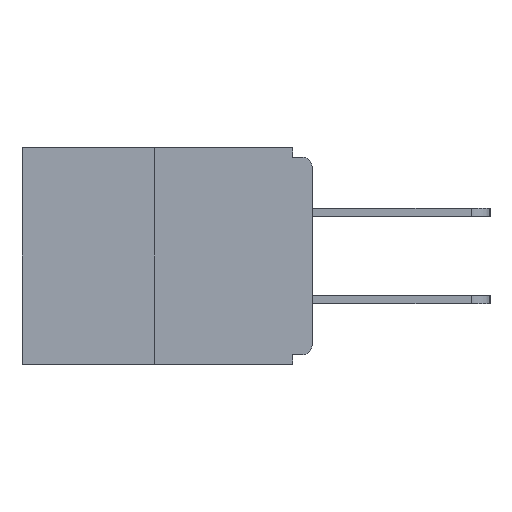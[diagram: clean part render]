
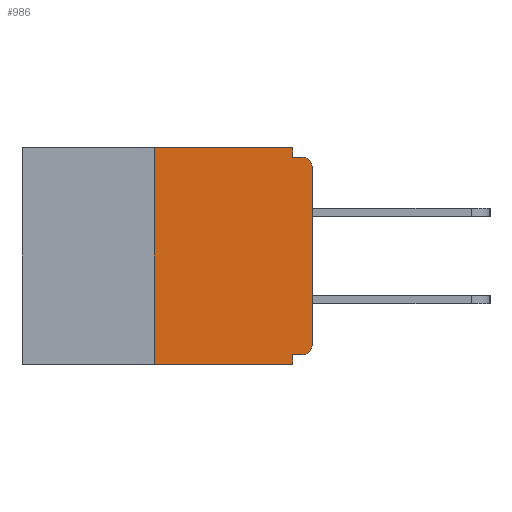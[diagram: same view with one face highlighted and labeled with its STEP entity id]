
A CAD part, left-side view. The second image highlights one B-rep face of the part: STEP entity #986.
In plain terms, the highlighted planar face has unit normal (-1, 0, 0).
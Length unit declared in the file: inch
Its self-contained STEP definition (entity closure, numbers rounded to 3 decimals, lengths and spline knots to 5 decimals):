
#679 = CARTESIAN_POINT ( 'NONE',  ( 0., 0., -0.328 ) ) ;
#821 = VECTOR ( 'NONE', #8570, 39.37008 ) ;
#969 = EDGE_CURVE ( 'NONE', #13510, #16980, #17780, .T. ) ;
#986 = ADVANCED_FACE ( 'NONE', ( #7331 ), #12792, .F. ) ;
#1070 = ORIENTED_EDGE ( 'NONE', *, *, #7644, .F. ) ;
#1169 = LINE ( 'NONE', #15121, #13582 ) ;
#1217 = CARTESIAN_POINT ( 'NONE',  ( 0., 0., -0.03 ) ) ;
#1364 = DIRECTION ( 'NONE',  ( 0., 0., -1. ) ) ;
#1931 = DIRECTION ( 'NONE',  ( 0., 0., 1. ) ) ;
#2120 = EDGE_CURVE ( 'NONE', #4434, #15515, #15768, .T. ) ;
#2386 = DIRECTION ( 'NONE',  ( 0., -1., 0. ) ) ;
#2391 = LINE ( 'NONE', #17080, #9612 ) ;
#3064 = ORIENTED_EDGE ( 'NONE', *, *, #12847, .T. ) ;
#3163 = DIRECTION ( 'NONE',  ( 0., -1., 0. ) ) ;
#3590 = EDGE_CURVE ( 'NONE', #17871, #13692, #2391, .T. ) ;
#3613 = ORIENTED_EDGE ( 'NONE', *, *, #2120, .F. ) ;
#3730 = CARTESIAN_POINT ( 'NONE',  ( 0., 0., -0.015 ) ) ;
#3843 = DIRECTION ( 'NONE',  ( 0., 0., -1. ) ) ;
#3907 = CARTESIAN_POINT ( 'NONE',  ( 0., 0.015, -0.313 ) ) ;
#3919 = ORIENTED_EDGE ( 'NONE', *, *, #17432, .F. ) ;
#3928 = DIRECTION ( 'NONE',  ( 0., 0., -1. ) ) ;
#4128 = ORIENTED_EDGE ( 'NONE', *, *, #14534, .T. ) ;
#4434 = VERTEX_POINT ( 'NONE', #6951 ) ;
#4508 = CARTESIAN_POINT ( 'NONE',  ( 0., 0.46, 0. ) ) ;
#5142 = AXIS2_PLACEMENT_3D ( 'NONE', #3907, #13659, #3843 ) ;
#5279 = CARTESIAN_POINT ( 'NONE',  ( 0., 0.031, -0.328 ) ) ;
#5330 = LINE ( 'NONE', #15481, #10997 ) ;
#5523 = VERTEX_POINT ( 'NONE', #10822 ) ;
#6031 = CARTESIAN_POINT ( 'NONE',  ( 0., 0.25, -0.343 ) ) ;
#6951 = CARTESIAN_POINT ( 'NONE',  ( 0., 0.031, -0.015 ) ) ;
#7331 = FACE_OUTER_BOUND ( 'NONE', #8461, .T. ) ;
#7545 = VECTOR ( 'NONE', #17024, 39.37008 ) ;
#7644 = EDGE_CURVE ( 'NONE', #12853, #13510, #14135, .T. ) ;
#7843 = ORIENTED_EDGE ( 'NONE', *, *, #3590, .F. ) ;
#8461 = EDGE_LOOP ( 'NONE', ( #7843, #11619, #3064, #9568, #1070, #9925, #4128, #17233, #3613, #3919 ) ) ;
#8570 = DIRECTION ( 'NONE',  ( 0., -1., 0. ) ) ;
#8738 = DIRECTION ( 'NONE',  ( 0., 0., -1. ) ) ;
#8933 = VERTEX_POINT ( 'NONE', #1217 ) ;
#9047 = CIRCLE ( 'NONE', #10763, 0.015 ) ;
#9240 = CIRCLE ( 'NONE', #5142, 0.015 ) ;
#9568 = ORIENTED_EDGE ( 'NONE', *, *, #969, .F. ) ;
#9612 = VECTOR ( 'NONE', #3163, 39.37008 ) ;
#9770 = LINE ( 'NONE', #12065, #821 ) ;
#9925 = ORIENTED_EDGE ( 'NONE', *, *, #15788, .T. ) ;
#9928 = CARTESIAN_POINT ( 'NONE',  ( 0., 0.031, -0.343 ) ) ;
#10028 = CARTESIAN_POINT ( 'NONE',  ( 0., 0.015, -0.015 ) ) ;
#10105 = CARTESIAN_POINT ( 'NONE',  ( 0., 0., 0. ) ) ;
#10763 = AXIS2_PLACEMENT_3D ( 'NONE', #13932, #16737, #3928 ) ;
#10822 = CARTESIAN_POINT ( 'NONE',  ( 0., 0., -0.313 ) ) ;
#10856 = CARTESIAN_POINT ( 'NONE',  ( 0., 0.25, 0. ) ) ;
#10997 = VECTOR ( 'NONE', #11327, 39.37008 ) ;
#11173 = CARTESIAN_POINT ( 'NONE',  ( 0., 0.031, 0. ) ) ;
#11327 = DIRECTION ( 'NONE',  ( 0., 0., 1. ) ) ;
#11619 = ORIENTED_EDGE ( 'NONE', *, *, #14103, .F. ) ;
#11844 = VECTOR ( 'NONE', #2386, 39.37008 ) ;
#12065 = CARTESIAN_POINT ( 'NONE',  ( 0., 0.46, -0.343 ) ) ;
#12792 = PLANE ( 'NONE',  #13249 ) ;
#12820 = VECTOR ( 'NONE', #13079, 39.37008 ) ;
#12847 = EDGE_CURVE ( 'NONE', #15111, #16980, #9770, .T. ) ;
#12853 = VERTEX_POINT ( 'NONE', #15317 ) ;
#12915 = DIRECTION ( 'NONE',  ( 1., 0., 0. ) ) ;
#13079 = DIRECTION ( 'NONE',  ( 0., 1., 0. ) ) ;
#13249 = AXIS2_PLACEMENT_3D ( 'NONE', #4508, #12915, #8738 ) ;
#13510 = VERTEX_POINT ( 'NONE', #5279 ) ;
#13582 = VECTOR ( 'NONE', #1364, 39.37008 ) ;
#13602 = LINE ( 'NONE', #10105, #17767 ) ;
#13659 = DIRECTION ( 'NONE',  ( -1., 0., 0. ) ) ;
#13692 = VERTEX_POINT ( 'NONE', #11173 ) ;
#13932 = CARTESIAN_POINT ( 'NONE',  ( 0., 0.015, -0.03 ) ) ;
#14080 = CARTESIAN_POINT ( 'NONE',  ( 0., 0.031, -0.343 ) ) ;
#14103 = EDGE_CURVE ( 'NONE', #15111, #17871, #5330, .T. ) ;
#14135 = LINE ( 'NONE', #679, #12820 ) ;
#14534 = EDGE_CURVE ( 'NONE', #5523, #8933, #13602, .T. ) ;
#15111 = VERTEX_POINT ( 'NONE', #6031 ) ;
#15121 = CARTESIAN_POINT ( 'NONE',  ( 0., 0.031, 0. ) ) ;
#15317 = CARTESIAN_POINT ( 'NONE',  ( 0., 0.015, -0.328 ) ) ;
#15353 = EDGE_CURVE ( 'NONE', #8933, #15515, #9047, .T. ) ;
#15481 = CARTESIAN_POINT ( 'NONE',  ( 0., 0.25, 0. ) ) ;
#15515 = VERTEX_POINT ( 'NONE', #10028 ) ;
#15768 = LINE ( 'NONE', #3730, #11844 ) ;
#15788 = EDGE_CURVE ( 'NONE', #12853, #5523, #9240, .T. ) ;
#16737 = DIRECTION ( 'NONE',  ( -1., 0., 0. ) ) ;
#16980 = VERTEX_POINT ( 'NONE', #9928 ) ;
#17024 = DIRECTION ( 'NONE',  ( 0., 0., -1. ) ) ;
#17080 = CARTESIAN_POINT ( 'NONE',  ( 0., 0.46, 0. ) ) ;
#17233 = ORIENTED_EDGE ( 'NONE', *, *, #15353, .T. ) ;
#17432 = EDGE_CURVE ( 'NONE', #13692, #4434, #1169, .T. ) ;
#17767 = VECTOR ( 'NONE', #1931, 39.37008 ) ;
#17780 = LINE ( 'NONE', #14080, #7545 ) ;
#17871 = VERTEX_POINT ( 'NONE', #10856 ) ;
